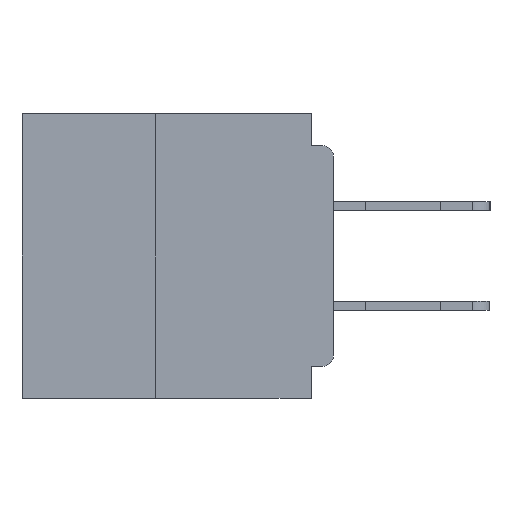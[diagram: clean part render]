
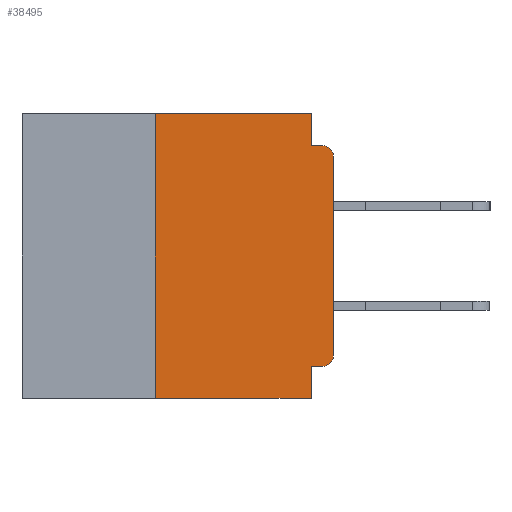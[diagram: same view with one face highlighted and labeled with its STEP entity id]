
A CAD part, left-side view. The second image highlights one B-rep face of the part: STEP entity #38495.
In plain terms, the highlighted planar face has unit normal (-1, 0, 0).
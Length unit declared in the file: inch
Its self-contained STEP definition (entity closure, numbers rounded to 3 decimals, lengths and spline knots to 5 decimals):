
#976 = CARTESIAN_POINT ( 'NONE',  ( 0., 0., 0. ) ) ;
#1687 = EDGE_CURVE ( 'NONE', #14276, #23088, #12071, .T. ) ;
#3844 = CARTESIAN_POINT ( 'NONE',  ( 0., 0.25, 0. ) ) ;
#3916 = EDGE_CURVE ( 'NONE', #25329, #28100, #6641, .T. ) ;
#3919 = VERTEX_POINT ( 'NONE', #4102 ) ;
#3998 = VECTOR ( 'NONE', #20312, 39.37008 ) ;
#4102 = CARTESIAN_POINT ( 'NONE',  ( 0., 0.031, -0.045 ) ) ;
#4239 = ORIENTED_EDGE ( 'NONE', *, *, #16087, .F. ) ;
#4376 = CARTESIAN_POINT ( 'NONE',  ( 0., 0.437, -0.4 ) ) ;
#5866 = LINE ( 'NONE', #4376, #37053 ) ;
#6641 = LINE ( 'NONE', #976, #13817 ) ;
#6743 = CARTESIAN_POINT ( 'NONE',  ( 0., 0.015, -0.34 ) ) ;
#6811 = DIRECTION ( 'NONE',  ( 0., 0., -1. ) ) ;
#7194 = DIRECTION ( 'NONE',  ( -1., 0., 0. ) ) ;
#7582 = DIRECTION ( 'NONE',  ( 0., -1., 0. ) ) ;
#7834 = EDGE_CURVE ( 'NONE', #28100, #26150, #22622, .T. ) ;
#7911 = VECTOR ( 'NONE', #7582, 39.37008 ) ;
#8998 = AXIS2_PLACEMENT_3D ( 'NONE', #15697, #36769, #18681 ) ;
#9817 = DIRECTION ( 'NONE',  ( 0., 0., -1. ) ) ;
#10229 = VECTOR ( 'NONE', #34658, 39.37008 ) ;
#11171 = LINE ( 'NONE', #31635, #10229 ) ;
#12071 = LINE ( 'NONE', #21525, #3998 ) ;
#12705 = CARTESIAN_POINT ( 'NONE',  ( 0., 0., -0.34 ) ) ;
#13539 = DIRECTION ( 'NONE',  ( 0., -1., 0. ) ) ;
#13797 = EDGE_CURVE ( 'NONE', #15254, #3919, #20306, .T. ) ;
#13817 = VECTOR ( 'NONE', #25294, 39.37008 ) ;
#14276 = VERTEX_POINT ( 'NONE', #21307 ) ;
#14347 = VECTOR ( 'NONE', #16256, 39.37008 ) ;
#15010 = LINE ( 'NONE', #22628, #7911 ) ;
#15254 = VERTEX_POINT ( 'NONE', #15304 ) ;
#15304 = CARTESIAN_POINT ( 'NONE',  ( 0., 0.031, 0. ) ) ;
#15697 = CARTESIAN_POINT ( 'NONE',  ( 0., 0.437, 0. ) ) ;
#16087 = EDGE_CURVE ( 'NONE', #3919, #26150, #15010, .T. ) ;
#16256 = DIRECTION ( 'NONE',  ( 0., -1., 0. ) ) ;
#16272 = VERTEX_POINT ( 'NONE', #26638 ) ;
#17735 = CIRCLE ( 'NONE', #28438, 0.015 ) ;
#18681 = DIRECTION ( 'NONE',  ( 0., 0., -1. ) ) ;
#19205 = CARTESIAN_POINT ( 'NONE',  ( 0., 0.015, -0.355 ) ) ;
#19261 = CARTESIAN_POINT ( 'NONE',  ( 0., 0.437, 0. ) ) ;
#19529 = LINE ( 'NONE', #34296, #32806 ) ;
#19877 = ORIENTED_EDGE ( 'NONE', *, *, #26660, .F. ) ;
#20306 = LINE ( 'NONE', #24956, #39096 ) ;
#20312 = DIRECTION ( 'NONE',  ( 0., 0., 1. ) ) ;
#20391 = CARTESIAN_POINT ( 'NONE',  ( 0., 0., -0.06 ) ) ;
#21307 = CARTESIAN_POINT ( 'NONE',  ( 0., 0.25, -0.4 ) ) ;
#21525 = CARTESIAN_POINT ( 'NONE',  ( 0., 0.25, -0.4 ) ) ;
#22245 = DIRECTION ( 'NONE',  ( 0., 1., 0. ) ) ;
#22622 = CIRCLE ( 'NONE', #23579, 0.015 ) ;
#22628 = CARTESIAN_POINT ( 'NONE',  ( 0., 0., -0.045 ) ) ;
#23051 = CARTESIAN_POINT ( 'NONE',  ( 0., 0.031, -0.355 ) ) ;
#23088 = VERTEX_POINT ( 'NONE', #3844 ) ;
#23579 = AXIS2_PLACEMENT_3D ( 'NONE', #25348, #7194, #28383 ) ;
#24278 = VERTEX_POINT ( 'NONE', #23051 ) ;
#24956 = CARTESIAN_POINT ( 'NONE',  ( 0., 0.031, 0. ) ) ;
#25294 = DIRECTION ( 'NONE',  ( 0., 0., 1. ) ) ;
#25329 = VERTEX_POINT ( 'NONE', #12705 ) ;
#25348 = CARTESIAN_POINT ( 'NONE',  ( 0., 0.015, -0.06 ) ) ;
#26103 = VERTEX_POINT ( 'NONE', #19205 ) ;
#26150 = VERTEX_POINT ( 'NONE', #28652 ) ;
#26638 = CARTESIAN_POINT ( 'NONE',  ( 0., 0.031, -0.4 ) ) ;
#26660 = EDGE_CURVE ( 'NONE', #24278, #16272, #11171, .T. ) ;
#27776 = ORIENTED_EDGE ( 'NONE', *, *, #1687, .F. ) ;
#27881 = ORIENTED_EDGE ( 'NONE', *, *, #34289, .T. ) ;
#27944 = DIRECTION ( 'NONE',  ( -1., 0., 0. ) ) ;
#28100 = VERTEX_POINT ( 'NONE', #20391 ) ;
#28383 = DIRECTION ( 'NONE',  ( 0., 0., -1. ) ) ;
#28438 = AXIS2_PLACEMENT_3D ( 'NONE', #6743, #27944, #9817 ) ;
#28652 = CARTESIAN_POINT ( 'NONE',  ( 0., 0.015, -0.045 ) ) ;
#28821 = ORIENTED_EDGE ( 'NONE', *, *, #13797, .F. ) ;
#28957 = ORIENTED_EDGE ( 'NONE', *, *, #35553, .F. ) ;
#29166 = EDGE_CURVE ( 'NONE', #23088, #15254, #38325, .T. ) ;
#29405 = ORIENTED_EDGE ( 'NONE', *, *, #29166, .F. ) ;
#30761 = PLANE ( 'NONE',  #8998 ) ;
#31635 = CARTESIAN_POINT ( 'NONE',  ( 0., 0.031, -0.4 ) ) ;
#32806 = VECTOR ( 'NONE', #22245, 39.37008 ) ;
#34289 = EDGE_CURVE ( 'NONE', #26103, #25329, #17735, .T. ) ;
#34296 = CARTESIAN_POINT ( 'NONE',  ( 0., 0., -0.355 ) ) ;
#34658 = DIRECTION ( 'NONE',  ( 0., 0., -1. ) ) ;
#35265 = ORIENTED_EDGE ( 'NONE', *, *, #3916, .T. ) ;
#35553 = EDGE_CURVE ( 'NONE', #26103, #24278, #19529, .T. ) ;
#35652 = FACE_OUTER_BOUND ( 'NONE', #38907, .T. ) ;
#36769 = DIRECTION ( 'NONE',  ( 1., 0., 0. ) ) ;
#37053 = VECTOR ( 'NONE', #13539, 39.37008 ) ;
#37570 = ORIENTED_EDGE ( 'NONE', *, *, #38224, .T. ) ;
#38224 = EDGE_CURVE ( 'NONE', #14276, #16272, #5866, .T. ) ;
#38325 = LINE ( 'NONE', #19261, #14347 ) ;
#38495 = ADVANCED_FACE ( 'NONE', ( #35652 ), #30761, .F. ) ;
#38871 = ORIENTED_EDGE ( 'NONE', *, *, #7834, .T. ) ;
#38907 = EDGE_LOOP ( 'NONE', ( #35265, #38871, #4239, #28821, #29405, #27776, #37570, #19877, #28957, #27881 ) ) ;
#39096 = VECTOR ( 'NONE', #6811, 39.37008 ) ;
